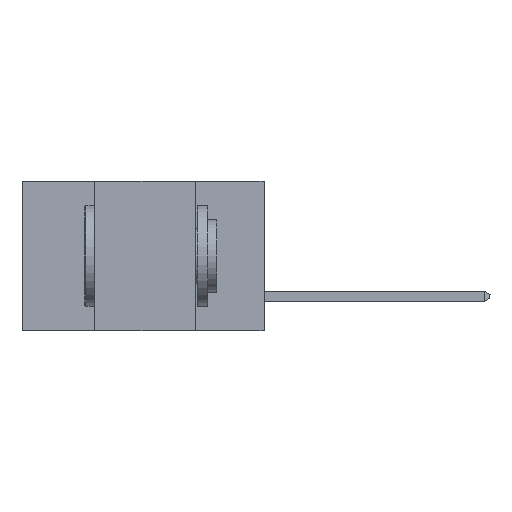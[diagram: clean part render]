
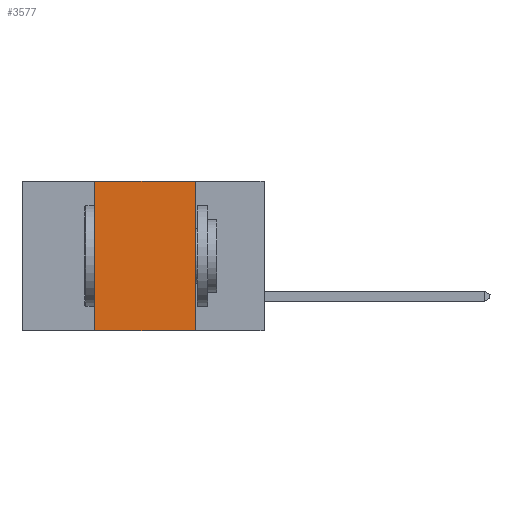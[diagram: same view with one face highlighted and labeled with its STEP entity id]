
A CAD part, left-side view. The second image highlights one B-rep face of the part: STEP entity #3577.
In plain terms, the highlighted planar face has unit normal (-1, 0, 0).
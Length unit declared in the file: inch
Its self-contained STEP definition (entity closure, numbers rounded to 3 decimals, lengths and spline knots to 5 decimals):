
#711 = DIRECTION ( 'NONE',  ( 0., 0., 1. ) ) ;
#975 = LINE ( 'NONE', #16448, #10391 ) ;
#990 = CARTESIAN_POINT ( 'NONE',  ( 0., 0.6, 0. ) ) ;
#2351 = PLANE ( 'NONE',  #8600 ) ;
#2991 = VECTOR ( 'NONE', #12980, 39.37008 ) ;
#3577 = ADVANCED_FACE ( 'NONE', ( #21609 ), #2351, .F. ) ;
#4443 = ORIENTED_EDGE ( 'NONE', *, *, #12888, .F. ) ;
#5907 = VERTEX_POINT ( 'NONE', #9706 ) ;
#5970 = CARTESIAN_POINT ( 'NONE',  ( 0., 0.17, -0.37 ) ) ;
#6271 = VERTEX_POINT ( 'NONE', #5970 ) ;
#7833 = CARTESIAN_POINT ( 'NONE',  ( 0., 0.17, -0.37 ) ) ;
#7943 = DIRECTION ( 'NONE',  ( 0., -1., 0. ) ) ;
#8092 = CARTESIAN_POINT ( 'NONE',  ( 0., 0.17, 0. ) ) ;
#8600 = AXIS2_PLACEMENT_3D ( 'NONE', #990, #16134, #14456 ) ;
#8972 = ORIENTED_EDGE ( 'NONE', *, *, #17923, .F. ) ;
#9515 = CARTESIAN_POINT ( 'NONE',  ( 0., 0.42, -0.37 ) ) ;
#9696 = EDGE_LOOP ( 'NONE', ( #8972, #10182, #4443, #22021 ) ) ;
#9706 = CARTESIAN_POINT ( 'NONE',  ( 0., 0.42, 0. ) ) ;
#10182 = ORIENTED_EDGE ( 'NONE', *, *, #17970, .F. ) ;
#10391 = VECTOR ( 'NONE', #14445, 39.37008 ) ;
#11926 = EDGE_CURVE ( 'NONE', #18060, #6271, #975, .T. ) ;
#11930 = VECTOR ( 'NONE', #7943, 39.37008 ) ;
#12759 = LINE ( 'NONE', #14787, #11930 ) ;
#12888 = EDGE_CURVE ( 'NONE', #18060, #5907, #21539, .T. ) ;
#12980 = DIRECTION ( 'NONE',  ( 0., 0., -1. ) ) ;
#14445 = DIRECTION ( 'NONE',  ( 0., -1., 0. ) ) ;
#14456 = DIRECTION ( 'NONE',  ( 0., 0., -1. ) ) ;
#14787 = CARTESIAN_POINT ( 'NONE',  ( 0., 0.6, 0. ) ) ;
#15070 = VECTOR ( 'NONE', #711, 39.37008 ) ;
#16134 = DIRECTION ( 'NONE',  ( 1., 0., 0. ) ) ;
#16448 = CARTESIAN_POINT ( 'NONE',  ( 0., 0.6, -0.37 ) ) ;
#17923 = EDGE_CURVE ( 'NONE', #21439, #6271, #19809, .T. ) ;
#17970 = EDGE_CURVE ( 'NONE', #5907, #21439, #12759, .T. ) ;
#18060 = VERTEX_POINT ( 'NONE', #9515 ) ;
#18174 = CARTESIAN_POINT ( 'NONE',  ( 0., 0.42, -0.37 ) ) ;
#19809 = LINE ( 'NONE', #7833, #2991 ) ;
#21439 = VERTEX_POINT ( 'NONE', #8092 ) ;
#21539 = LINE ( 'NONE', #18174, #15070 ) ;
#21609 = FACE_OUTER_BOUND ( 'NONE', #9696, .T. ) ;
#22021 = ORIENTED_EDGE ( 'NONE', *, *, #11926, .T. ) ;
